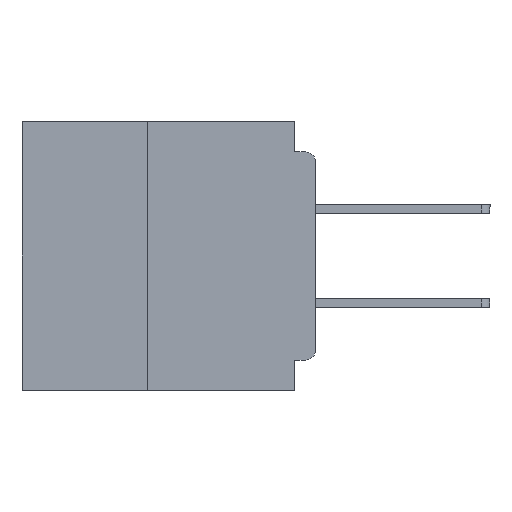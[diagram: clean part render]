
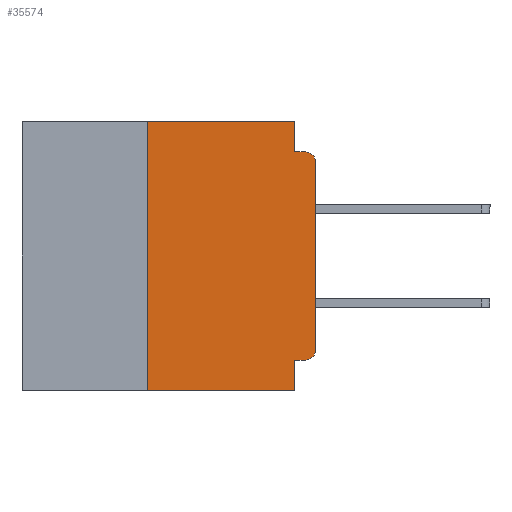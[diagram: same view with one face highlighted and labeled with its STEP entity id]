
A CAD part, left-side view. The second image highlights one B-rep face of the part: STEP entity #35574.
In plain terms, the highlighted planar face has unit normal (-1, 0, 0).
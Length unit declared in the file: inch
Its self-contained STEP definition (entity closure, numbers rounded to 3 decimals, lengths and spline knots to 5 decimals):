
#421 = VERTEX_POINT ( 'NONE', #33444 ) ;
#937 = DIRECTION ( 'NONE',  ( 0., 1., 0. ) ) ;
#1269 = VERTEX_POINT ( 'NONE', #2160 ) ;
#1800 = VECTOR ( 'NONE', #23319, 39.37008 ) ;
#2043 = EDGE_CURVE ( 'NONE', #20380, #7242, #3870, .T. ) ;
#2160 = CARTESIAN_POINT ( 'NONE',  ( 0., 0.015, -0.355 ) ) ;
#3870 = LINE ( 'NONE', #33255, #27656 ) ;
#5390 = CARTESIAN_POINT ( 'NONE',  ( 0., 0.015, -0.34 ) ) ;
#5534 = DIRECTION ( 'NONE',  ( 0., -1., 0. ) ) ;
#6627 = CARTESIAN_POINT ( 'NONE',  ( 0., 0.031, 0. ) ) ;
#7242 = VERTEX_POINT ( 'NONE', #50205 ) ;
#8519 = CARTESIAN_POINT ( 'NONE',  ( 0., 0., -0.34 ) ) ;
#8563 = AXIS2_PLACEMENT_3D ( 'NONE', #49090, #24028, #53277 ) ;
#8608 = CARTESIAN_POINT ( 'NONE',  ( 0., 0.25, -0.4 ) ) ;
#9691 = DIRECTION ( 'NONE',  ( 0., 0., -1. ) ) ;
#10890 = AXIS2_PLACEMENT_3D ( 'NONE', #47393, #22364, #51622 ) ;
#10940 = VECTOR ( 'NONE', #23586, 39.37008 ) ;
#12276 = ORIENTED_EDGE ( 'NONE', *, *, #29064, .F. ) ;
#13638 = CARTESIAN_POINT ( 'NONE',  ( 0., 0.031, -0.355 ) ) ;
#13719 = CARTESIAN_POINT ( 'NONE',  ( 0., 0.437, 0. ) ) ;
#15784 = EDGE_CURVE ( 'NONE', #47602, #421, #49216, .T. ) ;
#16237 = ORIENTED_EDGE ( 'NONE', *, *, #43764, .F. ) ;
#16259 = EDGE_CURVE ( 'NONE', #421, #7242, #20336, .T. ) ;
#17323 = DIRECTION ( 'NONE',  ( 0., 0., -1. ) ) ;
#19104 = CARTESIAN_POINT ( 'NONE',  ( 0., 0., 0. ) ) ;
#19442 = CARTESIAN_POINT ( 'NONE',  ( 0., 0.031, -0.4 ) ) ;
#19513 = ORIENTED_EDGE ( 'NONE', *, *, #31592, .F. ) ;
#19647 = EDGE_LOOP ( 'NONE', ( #24073, #29308, #40458, #19513, #12276, #23447, #37227, #16237, #27369, #52269 ) ) ;
#20336 = CIRCLE ( 'NONE', #10890, 0.015 ) ;
#20380 = VERTEX_POINT ( 'NONE', #44126 ) ;
#22364 = DIRECTION ( 'NONE',  ( -1., 0., 0. ) ) ;
#22604 = VERTEX_POINT ( 'NONE', #53807 ) ;
#23038 = CARTESIAN_POINT ( 'NONE',  ( 0., 0.25, -0.4 ) ) ;
#23319 = DIRECTION ( 'NONE',  ( 0., 0., 1. ) ) ;
#23447 = ORIENTED_EDGE ( 'NONE', *, *, #46621, .F. ) ;
#23522 = VERTEX_POINT ( 'NONE', #13638 ) ;
#23586 = DIRECTION ( 'NONE',  ( 0., 0., -1. ) ) ;
#24028 = DIRECTION ( 'NONE',  ( 1., 0., 0. ) ) ;
#24073 = ORIENTED_EDGE ( 'NONE', *, *, #15784, .T. ) ;
#24347 = VECTOR ( 'NONE', #937, 39.37008 ) ;
#27369 = ORIENTED_EDGE ( 'NONE', *, *, #47113, .F. ) ;
#27656 = VECTOR ( 'NONE', #33244, 39.37008 ) ;
#29064 = EDGE_CURVE ( 'NONE', #22604, #50943, #51505, .T. ) ;
#29214 = VECTOR ( 'NONE', #38823, 39.37008 ) ;
#29308 = ORIENTED_EDGE ( 'NONE', *, *, #16259, .T. ) ;
#29874 = CIRCLE ( 'NONE', #31495, 0.015 ) ;
#31495 = AXIS2_PLACEMENT_3D ( 'NONE', #5390, #34903, #9691 ) ;
#31592 = EDGE_CURVE ( 'NONE', #50943, #20380, #51580, .T. ) ;
#33244 = DIRECTION ( 'NONE',  ( 0., -1., 0. ) ) ;
#33255 = CARTESIAN_POINT ( 'NONE',  ( 0., 0., -0.045 ) ) ;
#33444 = CARTESIAN_POINT ( 'NONE',  ( 0., 0., -0.06 ) ) ;
#33448 = VERTEX_POINT ( 'NONE', #8608 ) ;
#34858 = CARTESIAN_POINT ( 'NONE',  ( 0., 0.437, -0.4 ) ) ;
#34903 = DIRECTION ( 'NONE',  ( -1., 0., 0. ) ) ;
#35574 = ADVANCED_FACE ( 'NONE', ( #36194 ), #36525, .F. ) ;
#36194 = FACE_OUTER_BOUND ( 'NONE', #19647, .T. ) ;
#36525 = PLANE ( 'NONE',  #8563 ) ;
#37227 = ORIENTED_EDGE ( 'NONE', *, *, #44867, .T. ) ;
#38183 = VECTOR ( 'NONE', #52297, 39.37008 ) ;
#38208 = CARTESIAN_POINT ( 'NONE',  ( 0., 0.031, 0. ) ) ;
#38823 = DIRECTION ( 'NONE',  ( 0., -1., 0. ) ) ;
#39861 = VERTEX_POINT ( 'NONE', #19442 ) ;
#40446 = VECTOR ( 'NONE', #17323, 39.37008 ) ;
#40458 = ORIENTED_EDGE ( 'NONE', *, *, #2043, .F. ) ;
#40794 = LINE ( 'NONE', #23038, #38183 ) ;
#43091 = LINE ( 'NONE', #52838, #10940 ) ;
#43764 = EDGE_CURVE ( 'NONE', #23522, #39861, #43091, .T. ) ;
#44126 = CARTESIAN_POINT ( 'NONE',  ( 0., 0.031, -0.045 ) ) ;
#44867 = EDGE_CURVE ( 'NONE', #33448, #39861, #52116, .T. ) ;
#46590 = LINE ( 'NONE', #51340, #24347 ) ;
#46621 = EDGE_CURVE ( 'NONE', #33448, #22604, #40794, .T. ) ;
#47113 = EDGE_CURVE ( 'NONE', #1269, #23522, #46590, .T. ) ;
#47393 = CARTESIAN_POINT ( 'NONE',  ( 0., 0.015, -0.06 ) ) ;
#47602 = VERTEX_POINT ( 'NONE', #8519 ) ;
#49090 = CARTESIAN_POINT ( 'NONE',  ( 0., 0.437, 0. ) ) ;
#49216 = LINE ( 'NONE', #19104, #1800 ) ;
#50205 = CARTESIAN_POINT ( 'NONE',  ( 0., 0.015, -0.045 ) ) ;
#50816 = VECTOR ( 'NONE', #5534, 39.37008 ) ;
#50943 = VERTEX_POINT ( 'NONE', #6627 ) ;
#51340 = CARTESIAN_POINT ( 'NONE',  ( 0., 0., -0.355 ) ) ;
#51505 = LINE ( 'NONE', #13719, #29214 ) ;
#51580 = LINE ( 'NONE', #38208, #40446 ) ;
#51622 = DIRECTION ( 'NONE',  ( 0., 0., -1. ) ) ;
#52116 = LINE ( 'NONE', #34858, #50816 ) ;
#52269 = ORIENTED_EDGE ( 'NONE', *, *, #54074, .T. ) ;
#52297 = DIRECTION ( 'NONE',  ( 0., 0., 1. ) ) ;
#52838 = CARTESIAN_POINT ( 'NONE',  ( 0., 0.031, -0.4 ) ) ;
#53277 = DIRECTION ( 'NONE',  ( 0., 0., -1. ) ) ;
#53807 = CARTESIAN_POINT ( 'NONE',  ( 0., 0.25, 0. ) ) ;
#54074 = EDGE_CURVE ( 'NONE', #1269, #47602, #29874, .T. ) ;
